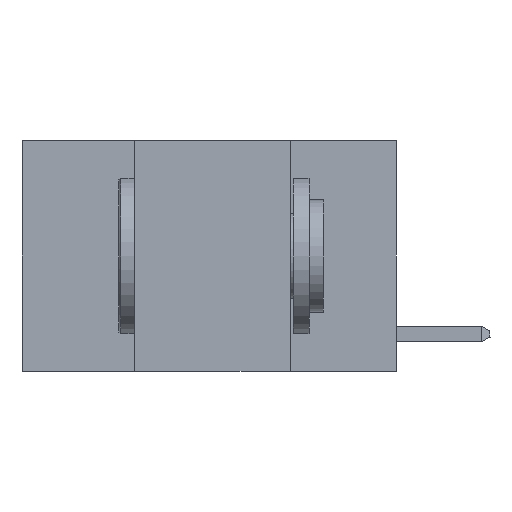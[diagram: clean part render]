
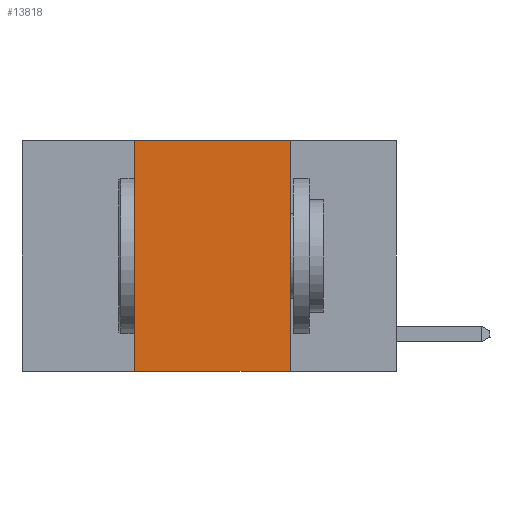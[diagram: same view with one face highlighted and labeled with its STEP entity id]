
A CAD part, left-side view. The second image highlights one B-rep face of the part: STEP entity #13818.
In plain terms, the highlighted planar face has unit normal (-1, 0, 0).
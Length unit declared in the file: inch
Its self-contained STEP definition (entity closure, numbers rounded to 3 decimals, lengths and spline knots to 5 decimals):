
#250 = VECTOR ( 'NONE', #11566, 39.37008 ) ;
#337 = CARTESIAN_POINT ( 'NONE',  ( 0., 0.17, 0. ) ) ;
#451 = VECTOR ( 'NONE', #17302, 39.37008 ) ;
#489 = DIRECTION ( 'NONE',  ( 0., 0., -1. ) ) ;
#838 = ORIENTED_EDGE ( 'NONE', *, *, #11913, .F. ) ;
#1064 = LINE ( 'NONE', #15485, #451 ) ;
#1591 = VERTEX_POINT ( 'NONE', #337 ) ;
#2062 = ORIENTED_EDGE ( 'NONE', *, *, #11801, .F. ) ;
#3259 = ORIENTED_EDGE ( 'NONE', *, *, #8265, .T. ) ;
#6053 = LINE ( 'NONE', #20988, #11693 ) ;
#7947 = LINE ( 'NONE', #15860, #12416 ) ;
#8265 = EDGE_CURVE ( 'NONE', #9480, #14075, #6053, .T. ) ;
#9480 = VERTEX_POINT ( 'NONE', #21649 ) ;
#10946 = LINE ( 'NONE', #20632, #250 ) ;
#11566 = DIRECTION ( 'NONE',  ( 0., -1., 0. ) ) ;
#11693 = VECTOR ( 'NONE', #15662, 39.37008 ) ;
#11801 = EDGE_CURVE ( 'NONE', #15275, #1591, #10946, .T. ) ;
#11866 = DIRECTION ( 'NONE',  ( 1., 0., 0. ) ) ;
#11913 = EDGE_CURVE ( 'NONE', #1591, #14075, #7947, .T. ) ;
#12134 = DIRECTION ( 'NONE',  ( 0., 0., -1. ) ) ;
#12416 = VECTOR ( 'NONE', #12134, 39.37008 ) ;
#12580 = CARTESIAN_POINT ( 'NONE',  ( 0., 0.17, -0.37 ) ) ;
#12697 = ORIENTED_EDGE ( 'NONE', *, *, #14451, .F. ) ;
#13676 = AXIS2_PLACEMENT_3D ( 'NONE', #22672, #11866, #489 ) ;
#13818 = ADVANCED_FACE ( 'NONE', ( #14698 ), #15512, .F. ) ;
#14075 = VERTEX_POINT ( 'NONE', #12580 ) ;
#14451 = EDGE_CURVE ( 'NONE', #9480, #15275, #1064, .T. ) ;
#14698 = FACE_OUTER_BOUND ( 'NONE', #19403, .T. ) ;
#15275 = VERTEX_POINT ( 'NONE', #19484 ) ;
#15485 = CARTESIAN_POINT ( 'NONE',  ( 0., 0.42, 0. ) ) ;
#15512 = PLANE ( 'NONE',  #13676 ) ;
#15662 = DIRECTION ( 'NONE',  ( 0., -1., 0. ) ) ;
#15860 = CARTESIAN_POINT ( 'NONE',  ( 0., 0.17, 0. ) ) ;
#17302 = DIRECTION ( 'NONE',  ( 0., 0., 1. ) ) ;
#19403 = EDGE_LOOP ( 'NONE', ( #838, #2062, #12697, #3259 ) ) ;
#19484 = CARTESIAN_POINT ( 'NONE',  ( 0., 0.42, 0. ) ) ;
#20632 = CARTESIAN_POINT ( 'NONE',  ( 0., 0.6, 0. ) ) ;
#20988 = CARTESIAN_POINT ( 'NONE',  ( 0., 0.6, -0.37 ) ) ;
#21649 = CARTESIAN_POINT ( 'NONE',  ( 0., 0.42, -0.37 ) ) ;
#22672 = CARTESIAN_POINT ( 'NONE',  ( 0., 0.6, 0. ) ) ;
